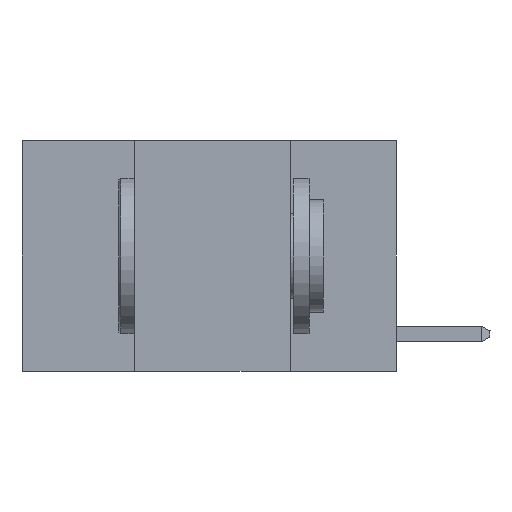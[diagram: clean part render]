
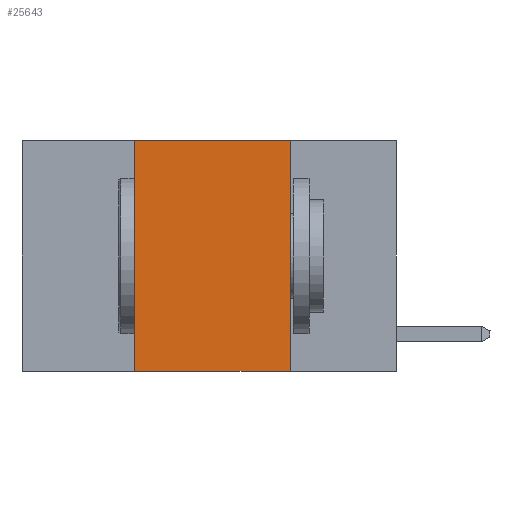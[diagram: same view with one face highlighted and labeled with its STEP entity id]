
A CAD part, left-side view. The second image highlights one B-rep face of the part: STEP entity #25643.
In plain terms, the highlighted planar face has unit normal (-1, 0, 0).
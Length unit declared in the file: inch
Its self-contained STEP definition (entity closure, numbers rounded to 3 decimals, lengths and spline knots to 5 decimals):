
#160 = CARTESIAN_POINT ( 'NONE',  ( 0., 0.17, 0. ) ) ;
#1981 = DIRECTION ( 'NONE',  ( 0., -1., 0. ) ) ;
#2605 = CARTESIAN_POINT ( 'NONE',  ( 0., 0.42, 0. ) ) ;
#2635 = CARTESIAN_POINT ( 'NONE',  ( 0., 0.42, 0. ) ) ;
#3496 = VERTEX_POINT ( 'NONE', #2635 ) ;
#4085 = VERTEX_POINT ( 'NONE', #17103 ) ;
#5045 = AXIS2_PLACEMENT_3D ( 'NONE', #20723, #15988, #18370 ) ;
#5825 = CARTESIAN_POINT ( 'NONE',  ( 0., 0.6, 0. ) ) ;
#6136 = CARTESIAN_POINT ( 'NONE',  ( 0., 0.6, -0.37 ) ) ;
#7754 = VERTEX_POINT ( 'NONE', #26294 ) ;
#7981 = ORIENTED_EDGE ( 'NONE', *, *, #19844, .T. ) ;
#8571 = FACE_OUTER_BOUND ( 'NONE', #28787, .T. ) ;
#8620 = CARTESIAN_POINT ( 'NONE',  ( 0., 0.17, 0. ) ) ;
#9299 = LINE ( 'NONE', #2605, #15275 ) ;
#10379 = VECTOR ( 'NONE', #23913, 39.37008 ) ;
#11883 = VERTEX_POINT ( 'NONE', #160 ) ;
#13389 = LINE ( 'NONE', #8620, #18692 ) ;
#14291 = ORIENTED_EDGE ( 'NONE', *, *, #21630, .F. ) ;
#15275 = VECTOR ( 'NONE', #27618, 39.37008 ) ;
#15988 = DIRECTION ( 'NONE',  ( 1., 0., 0. ) ) ;
#17103 = CARTESIAN_POINT ( 'NONE',  ( 0., 0.17, -0.37 ) ) ;
#17151 = ORIENTED_EDGE ( 'NONE', *, *, #23550, .F. ) ;
#17261 = VECTOR ( 'NONE', #1981, 39.37008 ) ;
#17268 = EDGE_CURVE ( 'NONE', #7754, #3496, #9299, .T. ) ;
#18370 = DIRECTION ( 'NONE',  ( 0., 0., -1. ) ) ;
#18692 = VECTOR ( 'NONE', #24466, 39.37008 ) ;
#19844 = EDGE_CURVE ( 'NONE', #7754, #4085, #27000, .T. ) ;
#20723 = CARTESIAN_POINT ( 'NONE',  ( 0., 0.6, 0. ) ) ;
#21630 = EDGE_CURVE ( 'NONE', #3496, #11883, #28193, .T. ) ;
#22933 = PLANE ( 'NONE',  #5045 ) ;
#23550 = EDGE_CURVE ( 'NONE', #11883, #4085, #13389, .T. ) ;
#23913 = DIRECTION ( 'NONE',  ( 0., -1., 0. ) ) ;
#24466 = DIRECTION ( 'NONE',  ( 0., 0., -1. ) ) ;
#25324 = ORIENTED_EDGE ( 'NONE', *, *, #17268, .F. ) ;
#25643 = ADVANCED_FACE ( 'NONE', ( #8571 ), #22933, .F. ) ;
#26294 = CARTESIAN_POINT ( 'NONE',  ( 0., 0.42, -0.37 ) ) ;
#27000 = LINE ( 'NONE', #6136, #17261 ) ;
#27618 = DIRECTION ( 'NONE',  ( 0., 0., 1. ) ) ;
#28193 = LINE ( 'NONE', #5825, #10379 ) ;
#28787 = EDGE_LOOP ( 'NONE', ( #17151, #14291, #25324, #7981 ) ) ;
